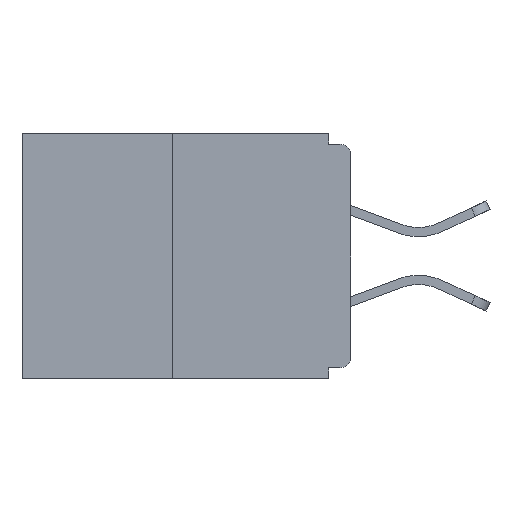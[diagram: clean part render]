
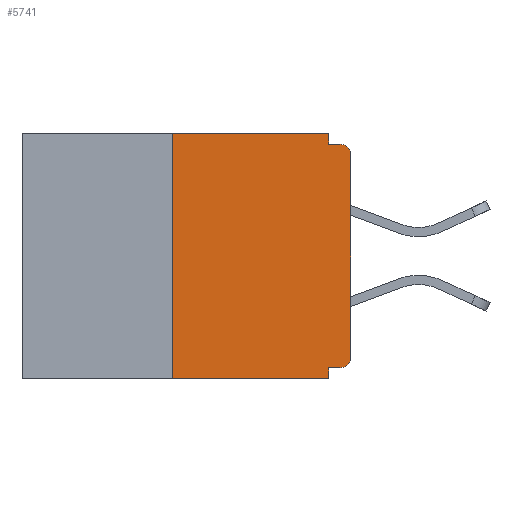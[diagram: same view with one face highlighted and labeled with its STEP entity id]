
A CAD part, left-side view. The second image highlights one B-rep face of the part: STEP entity #5741.
In plain terms, the highlighted planar face has unit normal (-1, 0, 0).
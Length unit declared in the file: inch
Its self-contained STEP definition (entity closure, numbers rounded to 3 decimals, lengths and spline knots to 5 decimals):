
#205 = CARTESIAN_POINT ( 'NONE',  ( 0., 0., 0. ) ) ;
#341 = FACE_OUTER_BOUND ( 'NONE', #4676, .T. ) ;
#994 = CARTESIAN_POINT ( 'NONE',  ( 0., 0.031, -0.015 ) ) ;
#1042 = DIRECTION ( 'NONE',  ( 0., -1., 0. ) ) ;
#1055 = DIRECTION ( 'NONE',  ( -1., 0., 0. ) ) ;
#1400 = CARTESIAN_POINT ( 'NONE',  ( 0., 0.015, -0.328 ) ) ;
#1526 = CIRCLE ( 'NONE', #5706, 0.015 ) ;
#1625 = CARTESIAN_POINT ( 'NONE',  ( 0., 0., -0.328 ) ) ;
#1691 = VERTEX_POINT ( 'NONE', #994 ) ;
#1837 = EDGE_CURVE ( 'NONE', #6105, #5241, #4880, .T. ) ;
#1981 = DIRECTION ( 'NONE',  ( 0., 0., 1. ) ) ;
#2118 = DIRECTION ( 'NONE',  ( 0., 0., -1. ) ) ;
#2248 = ORIENTED_EDGE ( 'NONE', *, *, #9600, .T. ) ;
#2380 = ORIENTED_EDGE ( 'NONE', *, *, #3371, .F. ) ;
#2627 = ORIENTED_EDGE ( 'NONE', *, *, #1837, .T. ) ;
#3296 = VECTOR ( 'NONE', #11966, 39.37008 ) ;
#3371 = EDGE_CURVE ( 'NONE', #6105, #5982, #7579, .T. ) ;
#3695 = CARTESIAN_POINT ( 'NONE',  ( 0., 0.031, -0.328 ) ) ;
#4092 = ORIENTED_EDGE ( 'NONE', *, *, #11650, .T. ) ;
#4426 = CARTESIAN_POINT ( 'NONE',  ( 0., 0.015, -0.313 ) ) ;
#4432 = LINE ( 'NONE', #205, #13082 ) ;
#4448 = CARTESIAN_POINT ( 'NONE',  ( 0., 0.015, -0.03 ) ) ;
#4504 = VECTOR ( 'NONE', #1042, 39.37008 ) ;
#4642 = VERTEX_POINT ( 'NONE', #3695 ) ;
#4676 = EDGE_LOOP ( 'NONE', ( #13440, #2380, #2627, #13071, #11239, #4092, #2248, #6260, #12217, #10720 ) ) ;
#4792 = EDGE_CURVE ( 'NONE', #5982, #11390, #6499, .T. ) ;
#4880 = LINE ( 'NONE', #9838, #7461 ) ;
#5192 = CARTESIAN_POINT ( 'NONE',  ( 0., 0.031, 0. ) ) ;
#5241 = VERTEX_POINT ( 'NONE', #13140 ) ;
#5338 = DIRECTION ( 'NONE',  ( 0., 0., -1. ) ) ;
#5706 = AXIS2_PLACEMENT_3D ( 'NONE', #4448, #10081, #9055 ) ;
#5741 = ADVANCED_FACE ( 'NONE', ( #341 ), #8534, .F. ) ;
#5982 = VERTEX_POINT ( 'NONE', #7051 ) ;
#6105 = VERTEX_POINT ( 'NONE', #13960 ) ;
#6260 = ORIENTED_EDGE ( 'NONE', *, *, #12557, .T. ) ;
#6499 = LINE ( 'NONE', #8334, #11370 ) ;
#6593 = LINE ( 'NONE', #8728, #4504 ) ;
#6630 = CIRCLE ( 'NONE', #10547, 0.015 ) ;
#6884 = DIRECTION ( 'NONE',  ( 0., 0., -1. ) ) ;
#7051 = CARTESIAN_POINT ( 'NONE',  ( 0., 0.25, 0. ) ) ;
#7459 = DIRECTION ( 'NONE',  ( 0., -1., 0. ) ) ;
#7461 = VECTOR ( 'NONE', #8625, 39.37008 ) ;
#7579 = LINE ( 'NONE', #12103, #9505 ) ;
#7616 = LINE ( 'NONE', #1625, #10926 ) ;
#7663 = EDGE_CURVE ( 'NONE', #9884, #4642, #7616, .T. ) ;
#8150 = VECTOR ( 'NONE', #6884, 39.37008 ) ;
#8334 = CARTESIAN_POINT ( 'NONE',  ( 0., 0.46, 0. ) ) ;
#8506 = LINE ( 'NONE', #13680, #8150 ) ;
#8534 = PLANE ( 'NONE',  #11331 ) ;
#8625 = DIRECTION ( 'NONE',  ( 0., -1., 0. ) ) ;
#8673 = DIRECTION ( 'NONE',  ( 1., 0., 0. ) ) ;
#8728 = CARTESIAN_POINT ( 'NONE',  ( 0., 0., -0.015 ) ) ;
#8956 = VERTEX_POINT ( 'NONE', #14181 ) ;
#9055 = DIRECTION ( 'NONE',  ( 0., 0., -1. ) ) ;
#9083 = CARTESIAN_POINT ( 'NONE',  ( 0., 0.031, 0. ) ) ;
#9331 = CARTESIAN_POINT ( 'NONE',  ( 0., 0., -0.03 ) ) ;
#9430 = DIRECTION ( 'NONE',  ( 0., 1., 0. ) ) ;
#9505 = VECTOR ( 'NONE', #1981, 39.37008 ) ;
#9600 = EDGE_CURVE ( 'NONE', #12096, #13831, #4432, .T. ) ;
#9838 = CARTESIAN_POINT ( 'NONE',  ( 0., 0.46, -0.343 ) ) ;
#9884 = VERTEX_POINT ( 'NONE', #1400 ) ;
#10081 = DIRECTION ( 'NONE',  ( -1., 0., 0. ) ) ;
#10547 = AXIS2_PLACEMENT_3D ( 'NONE', #4426, #1055, #2118 ) ;
#10720 = ORIENTED_EDGE ( 'NONE', *, *, #13301, .F. ) ;
#10926 = VECTOR ( 'NONE', #9430, 39.37008 ) ;
#11239 = ORIENTED_EDGE ( 'NONE', *, *, #7663, .F. ) ;
#11331 = AXIS2_PLACEMENT_3D ( 'NONE', #11978, #8673, #5338 ) ;
#11370 = VECTOR ( 'NONE', #7459, 39.37008 ) ;
#11390 = VERTEX_POINT ( 'NONE', #9083 ) ;
#11650 = EDGE_CURVE ( 'NONE', #9884, #12096, #6630, .T. ) ;
#11966 = DIRECTION ( 'NONE',  ( 0., 0., -1. ) ) ;
#11978 = CARTESIAN_POINT ( 'NONE',  ( 0., 0.46, 0. ) ) ;
#11999 = LINE ( 'NONE', #5192, #3296 ) ;
#12096 = VERTEX_POINT ( 'NONE', #13405 ) ;
#12103 = CARTESIAN_POINT ( 'NONE',  ( 0., 0.25, 0. ) ) ;
#12217 = ORIENTED_EDGE ( 'NONE', *, *, #13188, .F. ) ;
#12557 = EDGE_CURVE ( 'NONE', #13831, #8956, #1526, .T. ) ;
#12693 = EDGE_CURVE ( 'NONE', #4642, #5241, #8506, .T. ) ;
#13071 = ORIENTED_EDGE ( 'NONE', *, *, #12693, .F. ) ;
#13082 = VECTOR ( 'NONE', #13572, 39.37008 ) ;
#13140 = CARTESIAN_POINT ( 'NONE',  ( 0., 0.031, -0.343 ) ) ;
#13188 = EDGE_CURVE ( 'NONE', #1691, #8956, #6593, .T. ) ;
#13301 = EDGE_CURVE ( 'NONE', #11390, #1691, #11999, .T. ) ;
#13405 = CARTESIAN_POINT ( 'NONE',  ( 0., 0., -0.313 ) ) ;
#13440 = ORIENTED_EDGE ( 'NONE', *, *, #4792, .F. ) ;
#13572 = DIRECTION ( 'NONE',  ( 0., 0., 1. ) ) ;
#13680 = CARTESIAN_POINT ( 'NONE',  ( 0., 0.031, -0.343 ) ) ;
#13831 = VERTEX_POINT ( 'NONE', #9331 ) ;
#13960 = CARTESIAN_POINT ( 'NONE',  ( 0., 0.25, -0.343 ) ) ;
#14181 = CARTESIAN_POINT ( 'NONE',  ( 0., 0.015, -0.015 ) ) ;
